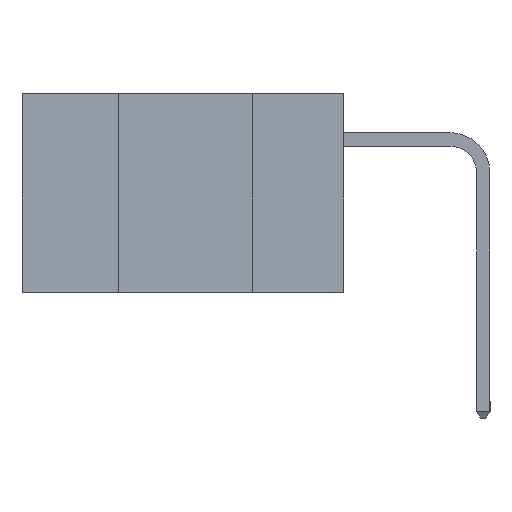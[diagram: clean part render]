
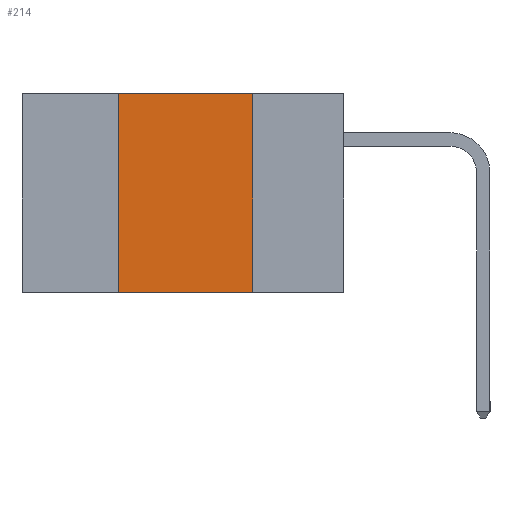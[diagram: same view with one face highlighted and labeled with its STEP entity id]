
A CAD part, left-side view. The second image highlights one B-rep face of the part: STEP entity #214.
In plain terms, the highlighted planar face has unit normal (-1, 0, 0).
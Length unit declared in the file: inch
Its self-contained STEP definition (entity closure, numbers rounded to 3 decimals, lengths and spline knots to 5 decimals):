
#214 = ADVANCED_FACE ( 'NONE', ( #2593 ), #4133, .F. ) ;
#256 = ORIENTED_EDGE ( 'NONE', *, *, #677, .F. ) ;
#677 = EDGE_CURVE ( 'NONE', #7217, #3306, #13796, .T. ) ;
#847 = EDGE_CURVE ( 'NONE', #6026, #3306, #11420, .T. ) ;
#885 = DIRECTION ( 'NONE',  ( 0., 0., -1. ) ) ;
#1179 = VECTOR ( 'NONE', #2887, 39.37008 ) ;
#1270 = CARTESIAN_POINT ( 'NONE',  ( 0., 0.17, 0. ) ) ;
#1700 = CARTESIAN_POINT ( 'NONE',  ( 0., 0.42, -0.37 ) ) ;
#2431 = EDGE_LOOP ( 'NONE', ( #256, #2621, #9964, #4776 ) ) ;
#2593 = FACE_OUTER_BOUND ( 'NONE', #2431, .T. ) ;
#2621 = ORIENTED_EDGE ( 'NONE', *, *, #13188, .F. ) ;
#2818 = DIRECTION ( 'NONE',  ( 0., 0., 1. ) ) ;
#2887 = DIRECTION ( 'NONE',  ( 0., -1., 0. ) ) ;
#2972 = CARTESIAN_POINT ( 'NONE',  ( 0., 0.6, -0.37 ) ) ;
#3306 = VERTEX_POINT ( 'NONE', #6085 ) ;
#4005 = CARTESIAN_POINT ( 'NONE',  ( 0., 0.42, -0.37 ) ) ;
#4133 = PLANE ( 'NONE',  #12530 ) ;
#4776 = ORIENTED_EDGE ( 'NONE', *, *, #847, .T. ) ;
#5634 = VECTOR ( 'NONE', #7350, 39.37008 ) ;
#5956 = EDGE_CURVE ( 'NONE', #6026, #6932, #10277, .T. ) ;
#6026 = VERTEX_POINT ( 'NONE', #4005 ) ;
#6085 = CARTESIAN_POINT ( 'NONE',  ( 0., 0.17, -0.37 ) ) ;
#6932 = VERTEX_POINT ( 'NONE', #13554 ) ;
#7217 = VERTEX_POINT ( 'NONE', #1270 ) ;
#7350 = DIRECTION ( 'NONE',  ( 0., -1., 0. ) ) ;
#7419 = DIRECTION ( 'NONE',  ( 1., 0., 0. ) ) ;
#8158 = DIRECTION ( 'NONE',  ( 0., 0., -1. ) ) ;
#8465 = CARTESIAN_POINT ( 'NONE',  ( 0., 0.6, 0. ) ) ;
#9936 = VECTOR ( 'NONE', #2818, 39.37008 ) ;
#9964 = ORIENTED_EDGE ( 'NONE', *, *, #5956, .F. ) ;
#10277 = LINE ( 'NONE', #1700, #9936 ) ;
#11392 = CARTESIAN_POINT ( 'NONE',  ( 0., 0.17, -0.37 ) ) ;
#11420 = LINE ( 'NONE', #2972, #5634 ) ;
#12427 = LINE ( 'NONE', #13722, #1179 ) ;
#12530 = AXIS2_PLACEMENT_3D ( 'NONE', #8465, #7419, #885 ) ;
#13188 = EDGE_CURVE ( 'NONE', #6932, #7217, #12427, .T. ) ;
#13461 = VECTOR ( 'NONE', #8158, 39.37008 ) ;
#13554 = CARTESIAN_POINT ( 'NONE',  ( 0., 0.42, 0. ) ) ;
#13722 = CARTESIAN_POINT ( 'NONE',  ( 0., 0.6, 0. ) ) ;
#13796 = LINE ( 'NONE', #11392, #13461 ) ;
